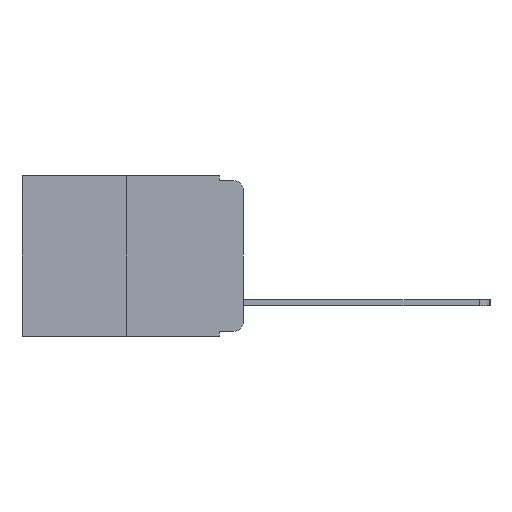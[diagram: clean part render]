
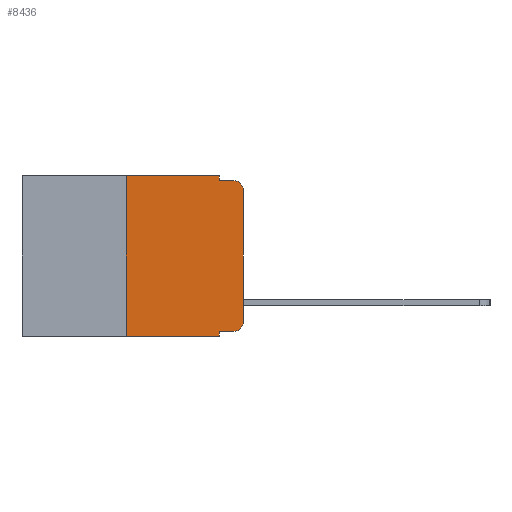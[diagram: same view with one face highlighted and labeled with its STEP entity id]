
A CAD part, left-side view. The second image highlights one B-rep face of the part: STEP entity #8436.
In plain terms, the highlighted planar face has unit normal (-1, 0, 0).
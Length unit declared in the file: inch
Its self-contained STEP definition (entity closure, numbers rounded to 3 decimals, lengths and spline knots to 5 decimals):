
#129 = VECTOR ( 'NONE', #9317, 39.37008 ) ;
#304 = VERTEX_POINT ( 'NONE', #9030 ) ;
#464 = CARTESIAN_POINT ( 'NONE',  ( 0., 0.473, 0. ) ) ;
#567 = CARTESIAN_POINT ( 'NONE',  ( 0., 0.051, -0.333 ) ) ;
#571 = LINE ( 'NONE', #1704, #5188 ) ;
#614 = DIRECTION ( 'NONE',  ( 0., 0., -1. ) ) ;
#1040 = DIRECTION ( 'NONE',  ( 0., 0., 1. ) ) ;
#1069 = CIRCLE ( 'NONE', #10042, 0.02 ) ;
#1234 = CARTESIAN_POINT ( 'NONE',  ( 0., 0.02, -0.01 ) ) ;
#1235 = VERTEX_POINT ( 'NONE', #567 ) ;
#1307 = DIRECTION ( 'NONE',  ( 1., 0., 0. ) ) ;
#1493 = EDGE_LOOP ( 'NONE', ( #10064, #4010, #7008, #7299, #7126, #7523, #7585, #6799, #3348, #1909 ) ) ;
#1704 = CARTESIAN_POINT ( 'NONE',  ( 0., 0.051, 0. ) ) ;
#1829 = AXIS2_PLACEMENT_3D ( 'NONE', #9444, #4334, #10251 ) ;
#1909 = ORIENTED_EDGE ( 'NONE', *, *, #8094, .T. ) ;
#2702 = LINE ( 'NONE', #4184, #129 ) ;
#2829 = VERTEX_POINT ( 'NONE', #10995 ) ;
#3214 = EDGE_CURVE ( 'NONE', #3495, #4053, #9623, .T. ) ;
#3313 = VERTEX_POINT ( 'NONE', #1234 ) ;
#3348 = ORIENTED_EDGE ( 'NONE', *, *, #9959, .T. ) ;
#3411 = EDGE_CURVE ( 'NONE', #7192, #4285, #7795, .T. ) ;
#3453 = VECTOR ( 'NONE', #6898, 39.37008 ) ;
#3495 = VERTEX_POINT ( 'NONE', #10336 ) ;
#3514 = VERTEX_POINT ( 'NONE', #9797 ) ;
#3841 = DIRECTION ( 'NONE',  ( 0., 0., 1. ) ) ;
#4010 = ORIENTED_EDGE ( 'NONE', *, *, #8551, .T. ) ;
#4053 = VERTEX_POINT ( 'NONE', #10285 ) ;
#4103 = CARTESIAN_POINT ( 'NONE',  ( 0., 0.473, 0. ) ) ;
#4139 = CARTESIAN_POINT ( 'NONE',  ( 0., 0.051, -0.01 ) ) ;
#4184 = CARTESIAN_POINT ( 'NONE',  ( 0., 0.051, -0.01 ) ) ;
#4285 = VERTEX_POINT ( 'NONE', #10289 ) ;
#4334 = DIRECTION ( 'NONE',  ( -1., 0., 0. ) ) ;
#4690 = CARTESIAN_POINT ( 'NONE',  ( 0., 0.25, 0. ) ) ;
#4810 = VECTOR ( 'NONE', #3841, 39.37008 ) ;
#5111 = EDGE_CURVE ( 'NONE', #10850, #3313, #2702, .T. ) ;
#5188 = VECTOR ( 'NONE', #7883, 39.37008 ) ;
#5344 = LINE ( 'NONE', #9773, #4810 ) ;
#5659 = CARTESIAN_POINT ( 'NONE',  ( 0., 0.051, -0.333 ) ) ;
#5833 = DIRECTION ( 'NONE',  ( 0., 0., -1. ) ) ;
#5886 = EDGE_CURVE ( 'NONE', #1235, #4285, #571, .T. ) ;
#5969 = LINE ( 'NONE', #5659, #10190 ) ;
#6073 = DIRECTION ( 'NONE',  ( -1., 0., 0. ) ) ;
#6279 = CIRCLE ( 'NONE', #1829, 0.02 ) ;
#6376 = CARTESIAN_POINT ( 'NONE',  ( 0., 0.051, 0. ) ) ;
#6690 = DIRECTION ( 'NONE',  ( 0., -1., 0. ) ) ;
#6725 = LINE ( 'NONE', #6376, #10839 ) ;
#6799 = ORIENTED_EDGE ( 'NONE', *, *, #5886, .F. ) ;
#6898 = DIRECTION ( 'NONE',  ( 0., -1., 0. ) ) ;
#6910 = CARTESIAN_POINT ( 'NONE',  ( 0., 0.473, -0.343 ) ) ;
#7008 = ORIENTED_EDGE ( 'NONE', *, *, #5111, .F. ) ;
#7126 = ORIENTED_EDGE ( 'NONE', *, *, #3214, .F. ) ;
#7192 = VERTEX_POINT ( 'NONE', #10395 ) ;
#7261 = DIRECTION ( 'NONE',  ( 0., 0., -1. ) ) ;
#7299 = ORIENTED_EDGE ( 'NONE', *, *, #7304, .F. ) ;
#7304 = EDGE_CURVE ( 'NONE', #4053, #10850, #6725, .T. ) ;
#7391 = VECTOR ( 'NONE', #6690, 39.37008 ) ;
#7523 = ORIENTED_EDGE ( 'NONE', *, *, #9294, .F. ) ;
#7585 = ORIENTED_EDGE ( 'NONE', *, *, #3411, .T. ) ;
#7770 = EDGE_CURVE ( 'NONE', #2829, #3514, #5344, .T. ) ;
#7795 = LINE ( 'NONE', #6910, #3453 ) ;
#7883 = DIRECTION ( 'NONE',  ( 0., 0., -1. ) ) ;
#8094 = EDGE_CURVE ( 'NONE', #304, #2829, #1069, .T. ) ;
#8436 = ADVANCED_FACE ( 'NONE', ( #10084 ), #10820, .F. ) ;
#8551 = EDGE_CURVE ( 'NONE', #3514, #3313, #6279, .T. ) ;
#8556 = AXIS2_PLACEMENT_3D ( 'NONE', #4103, #1307, #5833 ) ;
#9030 = CARTESIAN_POINT ( 'NONE',  ( 0., 0.02, -0.333 ) ) ;
#9052 = VECTOR ( 'NONE', #1040, 39.37008 ) ;
#9294 = EDGE_CURVE ( 'NONE', #7192, #3495, #11159, .T. ) ;
#9317 = DIRECTION ( 'NONE',  ( 0., -1., 0. ) ) ;
#9444 = CARTESIAN_POINT ( 'NONE',  ( 0., 0.02, -0.03 ) ) ;
#9623 = LINE ( 'NONE', #464, #7391 ) ;
#9773 = CARTESIAN_POINT ( 'NONE',  ( 0., 0., 0. ) ) ;
#9797 = CARTESIAN_POINT ( 'NONE',  ( 0., 0., -0.03 ) ) ;
#9874 = DIRECTION ( 'NONE',  ( 0., -1., 0. ) ) ;
#9959 = EDGE_CURVE ( 'NONE', #1235, #304, #5969, .T. ) ;
#10042 = AXIS2_PLACEMENT_3D ( 'NONE', #11033, #6073, #614 ) ;
#10064 = ORIENTED_EDGE ( 'NONE', *, *, #7770, .T. ) ;
#10084 = FACE_OUTER_BOUND ( 'NONE', #1493, .T. ) ;
#10190 = VECTOR ( 'NONE', #9874, 39.37008 ) ;
#10251 = DIRECTION ( 'NONE',  ( 0., 0., -1. ) ) ;
#10285 = CARTESIAN_POINT ( 'NONE',  ( 0., 0.051, 0. ) ) ;
#10289 = CARTESIAN_POINT ( 'NONE',  ( 0., 0.051, -0.343 ) ) ;
#10336 = CARTESIAN_POINT ( 'NONE',  ( 0., 0.25, 0. ) ) ;
#10395 = CARTESIAN_POINT ( 'NONE',  ( 0., 0.25, -0.343 ) ) ;
#10820 = PLANE ( 'NONE',  #8556 ) ;
#10839 = VECTOR ( 'NONE', #7261, 39.37008 ) ;
#10850 = VERTEX_POINT ( 'NONE', #4139 ) ;
#10995 = CARTESIAN_POINT ( 'NONE',  ( 0., 0., -0.313 ) ) ;
#11033 = CARTESIAN_POINT ( 'NONE',  ( 0., 0.02, -0.313 ) ) ;
#11159 = LINE ( 'NONE', #4690, #9052 ) ;
